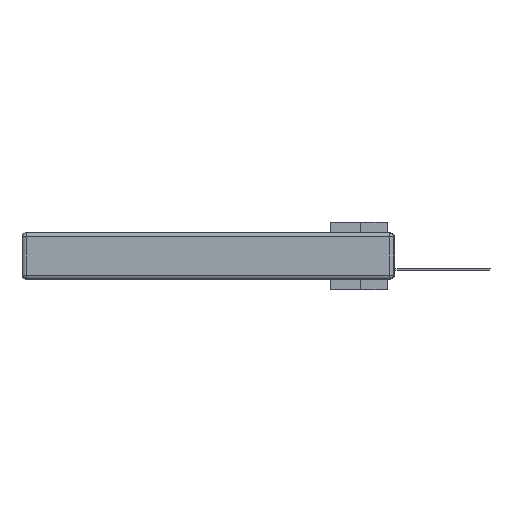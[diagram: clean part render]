
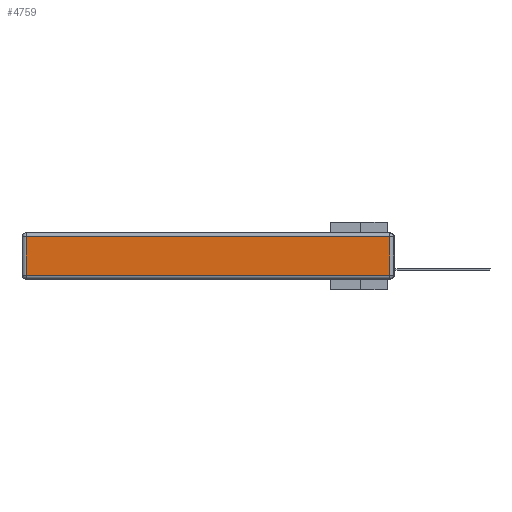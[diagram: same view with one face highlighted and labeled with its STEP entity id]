
A CAD part, left-side view. The second image highlights one B-rep face of the part: STEP entity #4759.
In plain terms, the highlighted planar face has unit normal (-1, 0, 0).
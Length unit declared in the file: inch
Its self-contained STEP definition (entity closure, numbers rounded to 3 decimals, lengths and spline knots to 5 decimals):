
#71 = CARTESIAN_POINT ( 'NONE',  ( 0., 2.75, -0.03 ) ) ;
#1783 = LINE ( 'NONE', #19242, #16486 ) ;
#1955 = DIRECTION ( 'NONE',  ( 0., 0., 1. ) ) ;
#2925 = DIRECTION ( 'NONE',  ( 0., 0., -1. ) ) ;
#3194 = CARTESIAN_POINT ( 'NONE',  ( 0., 0.03, -0.03 ) ) ;
#4759 = ADVANCED_FACE ( 'NONE', ( #28868 ), #18883, .T. ) ;
#4789 = VECTOR ( 'NONE', #22513, 39.37008 ) ;
#5618 = DIRECTION ( 'NONE',  ( 0., 0., 1. ) ) ;
#8272 = CARTESIAN_POINT ( 'NONE',  ( 0., 0., -0.343 ) ) ;
#9961 = VERTEX_POINT ( 'NONE', #3194 ) ;
#10604 = ORIENTED_EDGE ( 'NONE', *, *, #30129, .T. ) ;
#10975 = VECTOR ( 'NONE', #22870, 39.37008 ) ;
#11781 = VERTEX_POINT ( 'NONE', #29735 ) ;
#12694 = LINE ( 'NONE', #71, #4789 ) ;
#12864 = VECTOR ( 'NONE', #2925, 39.37008 ) ;
#15384 = LINE ( 'NONE', #22376, #10975 ) ;
#16486 = VECTOR ( 'NONE', #1955, 39.37008 ) ;
#18196 = ORIENTED_EDGE ( 'NONE', *, *, #20777, .T. ) ;
#18883 = PLANE ( 'NONE',  #24254 ) ;
#19242 = CARTESIAN_POINT ( 'NONE',  ( 0., 0.03, -0.343 ) ) ;
#20370 = CARTESIAN_POINT ( 'NONE',  ( 0., 2.72, -0.343 ) ) ;
#20538 = ORIENTED_EDGE ( 'NONE', *, *, #24320, .T. ) ;
#20777 = EDGE_CURVE ( 'NONE', #9961, #30833, #12694, .T. ) ;
#20971 = CARTESIAN_POINT ( 'NONE',  ( 0., 2.72, -0.313 ) ) ;
#21213 = EDGE_CURVE ( 'NONE', #11781, #9961, #1783, .T. ) ;
#22376 = CARTESIAN_POINT ( 'NONE',  ( 0., 0., -0.313 ) ) ;
#22513 = DIRECTION ( 'NONE',  ( 0., 1., 0. ) ) ;
#22870 = DIRECTION ( 'NONE',  ( 0., -1., 0. ) ) ;
#23548 = DIRECTION ( 'NONE',  ( -1., 0., 0. ) ) ;
#24254 = AXIS2_PLACEMENT_3D ( 'NONE', #8272, #23548, #5618 ) ;
#24320 = EDGE_CURVE ( 'NONE', #30833, #32535, #25188, .T. ) ;
#25188 = LINE ( 'NONE', #20370, #12864 ) ;
#26246 = EDGE_LOOP ( 'NONE', ( #10604, #31156, #18196, #20538 ) ) ;
#28868 = FACE_OUTER_BOUND ( 'NONE', #26246, .T. ) ;
#29735 = CARTESIAN_POINT ( 'NONE',  ( 0., 0.03, -0.313 ) ) ;
#30129 = EDGE_CURVE ( 'NONE', #32535, #11781, #15384, .T. ) ;
#30833 = VERTEX_POINT ( 'NONE', #31154 ) ;
#31154 = CARTESIAN_POINT ( 'NONE',  ( 0., 2.72, -0.03 ) ) ;
#31156 = ORIENTED_EDGE ( 'NONE', *, *, #21213, .T. ) ;
#32535 = VERTEX_POINT ( 'NONE', #20971 ) ;
